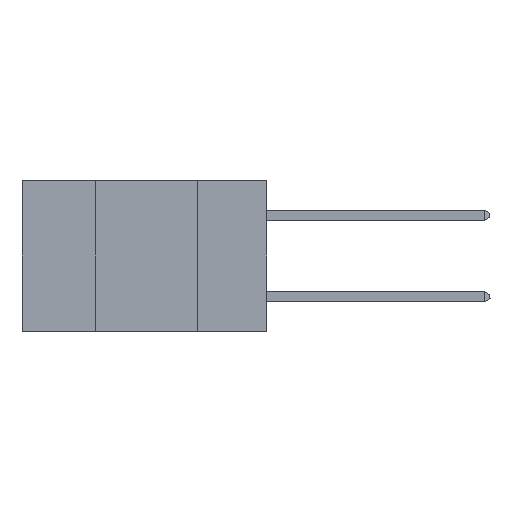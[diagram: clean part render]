
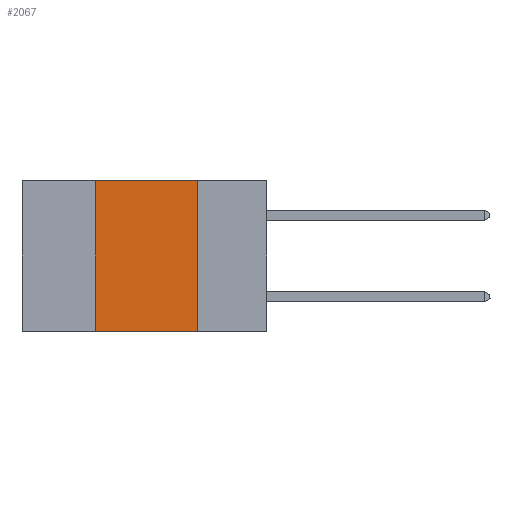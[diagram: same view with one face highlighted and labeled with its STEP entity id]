
A CAD part, left-side view. The second image highlights one B-rep face of the part: STEP entity #2067.
In plain terms, the highlighted planar face has unit normal (-1, 0, 0).
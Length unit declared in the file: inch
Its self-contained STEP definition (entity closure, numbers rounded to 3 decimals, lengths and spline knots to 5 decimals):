
#355 = DIRECTION ( 'NONE',  ( 0., -1., 0. ) ) ;
#490 = EDGE_LOOP ( 'NONE', ( #522, #8911, #618, #820 ) ) ;
#522 = ORIENTED_EDGE ( 'NONE', *, *, #3363, .F. ) ;
#618 = ORIENTED_EDGE ( 'NONE', *, *, #4079, .F. ) ;
#639 = VECTOR ( 'NONE', #355, 39.37008 ) ;
#820 = ORIENTED_EDGE ( 'NONE', *, *, #4806, .T. ) ;
#977 = VERTEX_POINT ( 'NONE', #6623 ) ;
#1087 = FACE_OUTER_BOUND ( 'NONE', #490, .T. ) ;
#2067 = ADVANCED_FACE ( 'NONE', ( #1087 ), #5496, .F. ) ;
#3170 = VERTEX_POINT ( 'NONE', #11358 ) ;
#3190 = CARTESIAN_POINT ( 'NONE',  ( 0., 0.6, 0. ) ) ;
#3363 = EDGE_CURVE ( 'NONE', #3170, #7824, #13042, .T. ) ;
#3956 = LINE ( 'NONE', #10865, #639 ) ;
#4079 = EDGE_CURVE ( 'NONE', #8254, #977, #9890, .T. ) ;
#4500 = EDGE_CURVE ( 'NONE', #977, #3170, #7527, .T. ) ;
#4806 = EDGE_CURVE ( 'NONE', #8254, #7824, #3956, .T. ) ;
#5444 = DIRECTION ( 'NONE',  ( 0., 0., -1. ) ) ;
#5449 = DIRECTION ( 'NONE',  ( 1., 0., 0. ) ) ;
#5496 = PLANE ( 'NONE',  #13028 ) ;
#5643 = CARTESIAN_POINT ( 'NONE',  ( 0., 0.6, 0. ) ) ;
#6623 = CARTESIAN_POINT ( 'NONE',  ( 0., 0.42, 0. ) ) ;
#7229 = VECTOR ( 'NONE', #10742, 39.37008 ) ;
#7527 = LINE ( 'NONE', #3190, #12562 ) ;
#7824 = VERTEX_POINT ( 'NONE', #12497 ) ;
#8254 = VERTEX_POINT ( 'NONE', #10314 ) ;
#8330 = DIRECTION ( 'NONE',  ( 0., -1., 0. ) ) ;
#8808 = DIRECTION ( 'NONE',  ( 0., 0., -1. ) ) ;
#8911 = ORIENTED_EDGE ( 'NONE', *, *, #4500, .F. ) ;
#9085 = CARTESIAN_POINT ( 'NONE',  ( 0., 0.17, 0. ) ) ;
#9712 = CARTESIAN_POINT ( 'NONE',  ( 0., 0.42, 0. ) ) ;
#9890 = LINE ( 'NONE', #9712, #7229 ) ;
#10314 = CARTESIAN_POINT ( 'NONE',  ( 0., 0.42, -0.37 ) ) ;
#10380 = VECTOR ( 'NONE', #8808, 39.37008 ) ;
#10742 = DIRECTION ( 'NONE',  ( 0., 0., 1. ) ) ;
#10865 = CARTESIAN_POINT ( 'NONE',  ( 0., 0.6, -0.37 ) ) ;
#11358 = CARTESIAN_POINT ( 'NONE',  ( 0., 0.17, 0. ) ) ;
#12497 = CARTESIAN_POINT ( 'NONE',  ( 0., 0.17, -0.37 ) ) ;
#12562 = VECTOR ( 'NONE', #8330, 39.37008 ) ;
#13028 = AXIS2_PLACEMENT_3D ( 'NONE', #5643, #5449, #5444 ) ;
#13042 = LINE ( 'NONE', #9085, #10380 ) ;
